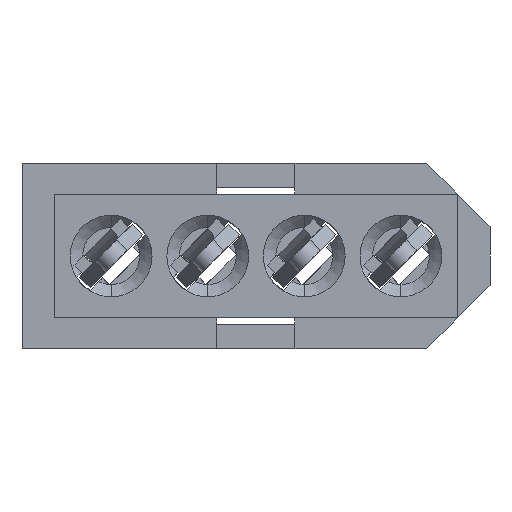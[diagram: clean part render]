
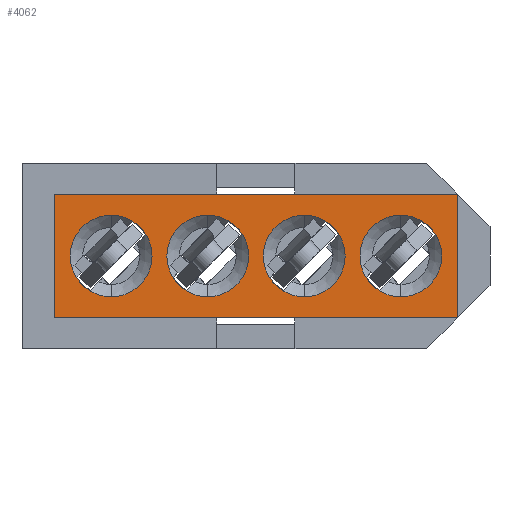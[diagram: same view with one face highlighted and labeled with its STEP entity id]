
A CAD part, front view. The second image highlights one B-rep face of the part: STEP entity #4062.
In plain terms, the highlighted planar face has unit normal (0, -1, 0).
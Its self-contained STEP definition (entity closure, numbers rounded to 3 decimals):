
#12 = CARTESIAN_POINT ( 'NONE',  ( 14.211, -12.7, -2.54 ) ) ;
#85 = AXIS2_PLACEMENT_3D ( 'NONE', #257, #4291, #4868 ) ;
#118 = CIRCLE ( 'NONE', #4342, 1.676 ) ;
#147 = VERTEX_POINT ( 'NONE', #2149 ) ;
#178 = AXIS2_PLACEMENT_3D ( 'NONE', #3941, #4533, #3316 ) ;
#257 = CARTESIAN_POINT ( 'NONE',  ( 11.887, -12.7, 0. ) ) ;
#268 = ORIENTED_EDGE ( 'NONE', *, *, #4525, .T. ) ;
#292 = CARTESIAN_POINT ( 'NONE',  ( -2.324, -12.7, -2.54 ) ) ;
#295 = EDGE_CURVE ( 'NONE', #4490, #147, #6916, .T. ) ;
#301 = FACE_BOUND ( 'NONE', #4571, .T. ) ;
#345 = CIRCLE ( 'NONE', #85, 1.676 ) ;
#390 = DIRECTION ( 'NONE',  ( 0., 1., 0. ) ) ;
#433 = VERTEX_POINT ( 'NONE', #2329 ) ;
#437 = LINE ( 'NONE', #1377, #1239 ) ;
#649 = FACE_BOUND ( 'NONE', #3492, .T. ) ;
#657 = DIRECTION ( 'NONE',  ( 0., 1., 0. ) ) ;
#703 = VERTEX_POINT ( 'NONE', #292 ) ;
#902 = DIRECTION ( 'NONE',  ( -1., 0., 0. ) ) ;
#906 = EDGE_CURVE ( 'NONE', #3820, #5042, #4975, .T. ) ;
#985 = ORIENTED_EDGE ( 'NONE', *, *, #906, .T. ) ;
#1075 = DIRECTION ( 'NONE',  ( 0., 0., 1. ) ) ;
#1090 = CARTESIAN_POINT ( 'NONE',  ( 3.962, -12.7, 0. ) ) ;
#1124 = AXIS2_PLACEMENT_3D ( 'NONE', #5676, #1658, #2842 ) ;
#1199 = EDGE_CURVE ( 'NONE', #6976, #7238, #6020, .T. ) ;
#1236 = LINE ( 'NONE', #5479, #1971 ) ;
#1239 = VECTOR ( 'NONE', #6390, 1000. ) ;
#1377 = CARTESIAN_POINT ( 'NONE',  ( -2.324, -12.7, 2.54 ) ) ;
#1636 = CARTESIAN_POINT ( 'NONE',  ( 3.962, -12.7, 1.676 ) ) ;
#1658 = DIRECTION ( 'NONE',  ( 0., 1., 0. ) ) ;
#1782 = ORIENTED_EDGE ( 'NONE', *, *, #4507, .F. ) ;
#1853 = AXIS2_PLACEMENT_3D ( 'NONE', #4300, #3168, #4873 ) ;
#1893 = CIRCLE ( 'NONE', #178, 1.676 ) ;
#1971 = VECTOR ( 'NONE', #902, 1000. ) ;
#2031 = EDGE_CURVE ( 'NONE', #7238, #6976, #118, .T. ) ;
#2072 = CARTESIAN_POINT ( 'NONE',  ( 11.887, -12.7, 0. ) ) ;
#2126 = EDGE_CURVE ( 'NONE', #5042, #3820, #2462, .T. ) ;
#2149 = CARTESIAN_POINT ( 'NONE',  ( 7.925, -12.7, -1.676 ) ) ;
#2173 = CARTESIAN_POINT ( 'NONE',  ( 7.925, -12.7, 1.676 ) ) ;
#2246 = ORIENTED_EDGE ( 'NONE', *, *, #295, .T. ) ;
#2251 = ORIENTED_EDGE ( 'NONE', *, *, #5347, .T. ) ;
#2329 = CARTESIAN_POINT ( 'NONE',  ( 14.211, -12.7, -2.54 ) ) ;
#2343 = EDGE_LOOP ( 'NONE', ( #1782, #5190, #5028, #2787 ) ) ;
#2356 = CARTESIAN_POINT ( 'NONE',  ( 0., -12.7, 1.676 ) ) ;
#2462 = CIRCLE ( 'NONE', #1124, 1.676 ) ;
#2750 = DIRECTION ( 'NONE',  ( 0., 0., 1. ) ) ;
#2787 = ORIENTED_EDGE ( 'NONE', *, *, #6306, .F. ) ;
#2842 = DIRECTION ( 'NONE',  ( 0., 0., 1. ) ) ;
#2912 = CARTESIAN_POINT ( 'NONE',  ( 0., -12.7, 0. ) ) ;
#3007 = DIRECTION ( 'NONE',  ( 0., 1., 0. ) ) ;
#3055 = EDGE_LOOP ( 'NONE', ( #3583, #7410 ) ) ;
#3168 = DIRECTION ( 'NONE',  ( 0., 1., 0. ) ) ;
#3267 = CARTESIAN_POINT ( 'NONE',  ( 0., -12.7, 0. ) ) ;
#3316 = DIRECTION ( 'NONE',  ( 0., 0., 1. ) ) ;
#3378 = EDGE_CURVE ( 'NONE', #4577, #433, #3413, .T. ) ;
#3413 = LINE ( 'NONE', #12, #5918 ) ;
#3415 = CARTESIAN_POINT ( 'NONE',  ( 11.887, -12.7, 1.676 ) ) ;
#3492 = EDGE_LOOP ( 'NONE', ( #2251, #6564 ) ) ;
#3518 = DIRECTION ( 'NONE',  ( 0., 1., 0. ) ) ;
#3583 = ORIENTED_EDGE ( 'NONE', *, *, #1199, .T. ) ;
#3700 = VERTEX_POINT ( 'NONE', #3415 ) ;
#3777 = CARTESIAN_POINT ( 'NONE',  ( 11.887, -12.7, -1.676 ) ) ;
#3820 = VERTEX_POINT ( 'NONE', #5231 ) ;
#3918 = CARTESIAN_POINT ( 'NONE',  ( 14.211, -12.7, 2.54 ) ) ;
#3941 = CARTESIAN_POINT ( 'NONE',  ( 7.925, -12.7, 0. ) ) ;
#4002 = EDGE_LOOP ( 'NONE', ( #2246, #268 ) ) ;
#4043 = DIRECTION ( 'NONE',  ( 0., 0., 1. ) ) ;
#4045 = CARTESIAN_POINT ( 'NONE',  ( -2.324, -12.7, 2.54 ) ) ;
#4062 = ADVANCED_FACE ( 'NONE', ( #649, #4685, #301, #6201, #5837 ), #4596, .F. ) ;
#4291 = DIRECTION ( 'NONE',  ( 0., 1., 0. ) ) ;
#4300 = CARTESIAN_POINT ( 'NONE',  ( 0., -12.7, 0. ) ) ;
#4309 = CIRCLE ( 'NONE', #7209, 1.676 ) ;
#4322 = DIRECTION ( 'NONE',  ( 0., 0., 1. ) ) ;
#4337 = AXIS2_PLACEMENT_3D ( 'NONE', #1090, #3518, #4043 ) ;
#4342 = AXIS2_PLACEMENT_3D ( 'NONE', #3267, #7302, #5583 ) ;
#4427 = EDGE_CURVE ( 'NONE', #5734, #3700, #4309, .T. ) ;
#4490 = VERTEX_POINT ( 'NONE', #2173 ) ;
#4507 = EDGE_CURVE ( 'NONE', #703, #6853, #5214, .T. ) ;
#4525 = EDGE_CURVE ( 'NONE', #147, #4490, #1893, .T. ) ;
#4533 = DIRECTION ( 'NONE',  ( 0., 1., 0. ) ) ;
#4571 = EDGE_LOOP ( 'NONE', ( #4630, #985 ) ) ;
#4577 = VERTEX_POINT ( 'NONE', #3918 ) ;
#4596 = PLANE ( 'NONE',  #7311 ) ;
#4630 = ORIENTED_EDGE ( 'NONE', *, *, #2126, .T. ) ;
#4634 = CARTESIAN_POINT ( 'NONE',  ( 7.925, -12.7, 0. ) ) ;
#4680 = DIRECTION ( 'NONE',  ( 0., 0., 1. ) ) ;
#4685 = FACE_BOUND ( 'NONE', #4002, .T. ) ;
#4868 = DIRECTION ( 'NONE',  ( 0., 0., 1. ) ) ;
#4873 = DIRECTION ( 'NONE',  ( 0., 0., 1. ) ) ;
#4975 = CIRCLE ( 'NONE', #4337, 1.676 ) ;
#5027 = VECTOR ( 'NONE', #2750, 1000. ) ;
#5028 = ORIENTED_EDGE ( 'NONE', *, *, #3378, .F. ) ;
#5042 = VERTEX_POINT ( 'NONE', #1636 ) ;
#5190 = ORIENTED_EDGE ( 'NONE', *, *, #5333, .F. ) ;
#5214 = LINE ( 'NONE', #5654, #5027 ) ;
#5231 = CARTESIAN_POINT ( 'NONE',  ( 3.962, -12.7, -1.676 ) ) ;
#5333 = EDGE_CURVE ( 'NONE', #433, #703, #1236, .T. ) ;
#5347 = EDGE_CURVE ( 'NONE', #3700, #5734, #345, .T. ) ;
#5479 = CARTESIAN_POINT ( 'NONE',  ( -2.324, -12.7, -2.54 ) ) ;
#5583 = DIRECTION ( 'NONE',  ( 0., 0., 1. ) ) ;
#5654 = CARTESIAN_POINT ( 'NONE',  ( -2.324, -12.7, -2.54 ) ) ;
#5676 = CARTESIAN_POINT ( 'NONE',  ( 3.962, -12.7, 0. ) ) ;
#5734 = VERTEX_POINT ( 'NONE', #3777 ) ;
#5837 = FACE_OUTER_BOUND ( 'NONE', #2343, .T. ) ;
#5918 = VECTOR ( 'NONE', #6850, 1000. ) ;
#6020 = CIRCLE ( 'NONE', #1853, 1.676 ) ;
#6042 = CARTESIAN_POINT ( 'NONE',  ( 0., -12.7, -1.676 ) ) ;
#6101 = AXIS2_PLACEMENT_3D ( 'NONE', #4634, #3007, #1075 ) ;
#6201 = FACE_BOUND ( 'NONE', #3055, .T. ) ;
#6306 = EDGE_CURVE ( 'NONE', #6853, #4577, #437, .T. ) ;
#6390 = DIRECTION ( 'NONE',  ( 1., 0., 0. ) ) ;
#6564 = ORIENTED_EDGE ( 'NONE', *, *, #4427, .T. ) ;
#6850 = DIRECTION ( 'NONE',  ( 0., 0., -1. ) ) ;
#6853 = VERTEX_POINT ( 'NONE', #4045 ) ;
#6916 = CIRCLE ( 'NONE', #6101, 1.676 ) ;
#6976 = VERTEX_POINT ( 'NONE', #2356 ) ;
#7209 = AXIS2_PLACEMENT_3D ( 'NONE', #2072, #390, #4322 ) ;
#7238 = VERTEX_POINT ( 'NONE', #6042 ) ;
#7302 = DIRECTION ( 'NONE',  ( 0., 1., 0. ) ) ;
#7311 = AXIS2_PLACEMENT_3D ( 'NONE', #2912, #657, #4680 ) ;
#7410 = ORIENTED_EDGE ( 'NONE', *, *, #2031, .T. ) ;
